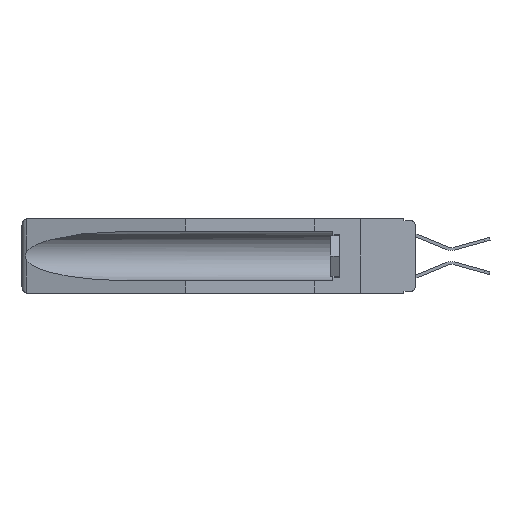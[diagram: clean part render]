
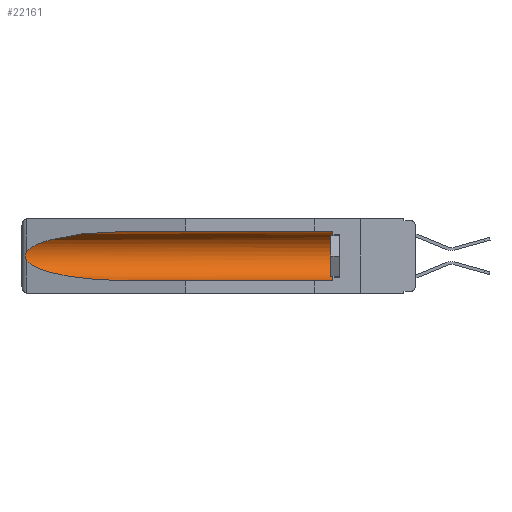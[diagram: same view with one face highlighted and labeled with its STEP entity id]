
A CAD part, left-side view. The second image highlights one B-rep face of the part: STEP entity #22161.
In plain terms, the highlighted cylindrical face has radius 2.857 mm (diameter 5.715 mm), a partial arc.
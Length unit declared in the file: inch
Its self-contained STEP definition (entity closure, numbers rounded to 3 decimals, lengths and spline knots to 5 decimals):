
#208 = ORIENTED_EDGE ( 'NONE', *, *, #10696, .T. ) ;
#1434 = CARTESIAN_POINT ( 'NONE',  ( 0.26654, 1.53092, -0.15636 ) ) ;
#1797 = EDGE_CURVE ( 'NONE', #14146, #15990, #14138, .T. ) ;
#2552 = B_SPLINE_CURVE_WITH_KNOTS ( 'NONE', 3,
 ( #2900, #11640, #1434, #8320, #16979, #10608, #3758, #6043, #16693, #10334 ),
 .UNSPECIFIED., .F., .F.,
 ( 4, 2, 2, 2, 4 ),
 ( 0., 0.00029, 0.00058, 0.00087, 0.00117 ),
 .UNSPECIFIED. ) ;
#2722 = EDGE_CURVE ( 'NONE', #16128, #4695, #17081, .T. ) ;
#2880 = AXIS2_PLACEMENT_3D ( 'NONE', #21203, #14833, #19715 ) ;
#2900 = CARTESIAN_POINT ( 'NONE',  ( 0.26537, 1.52718, -0.14972 ) ) ;
#3308 = CIRCLE ( 'NONE', #19399, 0.1125 ) ;
#3592 = CARTESIAN_POINT ( 'NONE',  ( 0.155, 1.07973, -0.059 ) ) ;
#3644 = FACE_OUTER_BOUND ( 'NONE', #17063, .T. ) ;
#3758 = CARTESIAN_POINT ( 'NONE',  ( 0.2673, 1.53269, -0.17917 ) ) ;
#4298 = CARTESIAN_POINT ( 'NONE',  ( 0.21114, 1.30732, -0.059 ) ) ;
#4695 = VERTEX_POINT ( 'NONE', #18701 ) ;
#5085 = CARTESIAN_POINT ( 'NONE',  ( 0.25451, 1.48313, -0.24835 ) ) ;
#5168 = VECTOR ( 'NONE', #14206, 39.37008 ) ;
#5821 = VERTEX_POINT ( 'NONE', #14071 ) ;
#6043 = CARTESIAN_POINT ( 'NONE',  ( 0.26655, 1.53094, -0.18657 ) ) ;
#6093 = LINE ( 'NONE', #22992, #11876 ) ;
#6508 = VERTEX_POINT ( 'NONE', #17469 ) ;
#7159 = DIRECTION ( 'NONE',  ( 0., 0., 1. ) ) ;
#7865 = LINE ( 'NONE', #25184, #5168 ) ;
#8320 = CARTESIAN_POINT ( 'NONE',  ( 0.2673, 1.5327, -0.16383 ) ) ;
#8718 = CARTESIAN_POINT ( 'NONE',  ( 0.155, 1.07973, -0.059 ) ) ;
#10334 = CARTESIAN_POINT ( 'NONE',  ( 0.26537, 1.52718, -0.19328 ) ) ;
#10608 = CARTESIAN_POINT ( 'NONE',  ( 0.2675, 1.53308, -0.17534 ) ) ;
#10696 = EDGE_CURVE ( 'NONE', #5821, #6508, #3308, .T. ) ;
#10762 = EDGE_CURVE ( 'NONE', #6508, #14146, #7865, .T. ) ;
#10884 = CYLINDRICAL_SURFACE ( 'NONE', #2880, 0.1125 ) ;
#11640 = CARTESIAN_POINT ( 'NONE',  ( 0.26597, 1.52961, -0.15275 ) ) ;
#11876 = VECTOR ( 'NONE', #21510, 39.37008 ) ;
#12680 = ORIENTED_EDGE ( 'NONE', *, *, #2722, .T. ) ;
#13232 = CARTESIAN_POINT ( 'NONE',  ( 0.26537, 1.52718, -0.14972 ) ) ;
#14071 = CARTESIAN_POINT ( 'NONE',  ( 0.155, 0.126, -0.284 ) ) ;
#14138 =( BOUNDED_CURVE ( )  B_SPLINE_CURVE ( 3, ( #8718, #4298, #24304, #21844 ),
 .UNSPECIFIED., .F., .F. ) 
 B_SPLINE_CURVE_WITH_KNOTS ( ( 4, 4 ),
 ( 4.71239, 6.08839 ),
 .UNSPECIFIED. ) 
 CURVE ( )  GEOMETRIC_REPRESENTATION_ITEM ( )  RATIONAL_B_SPLINE_CURVE ( ( 1., 0.848, 0.848, 1. ) ) 
 REPRESENTATION_ITEM ( '' )  );
#14146 = VERTEX_POINT ( 'NONE', #3592 ) ;
#14206 = DIRECTION ( 'NONE',  ( 0., 1., 0. ) ) ;
#14833 = DIRECTION ( 'NONE',  ( 0., 1., 0. ) ) ;
#15002 = EDGE_CURVE ( 'NONE', #15990, #16128, #2552, .T. ) ;
#15428 = CARTESIAN_POINT ( 'NONE',  ( 0.21114, 1.30732, -0.284 ) ) ;
#15990 = VERTEX_POINT ( 'NONE', #13232 ) ;
#16128 = VERTEX_POINT ( 'NONE', #24499 ) ;
#16693 = CARTESIAN_POINT ( 'NONE',  ( 0.26597, 1.5296, -0.19026 ) ) ;
#16979 = CARTESIAN_POINT ( 'NONE',  ( 0.2675, 1.53308, -0.16763 ) ) ;
#17063 = EDGE_LOOP ( 'NONE', ( #24952, #21673, #12680, #21898, #208, #23913 ) ) ;
#17081 =( BOUNDED_CURVE ( )  B_SPLINE_CURVE ( 3, ( #24814, #5085, #15428, #24243 ),
 .UNSPECIFIED., .F., .F. ) 
 B_SPLINE_CURVE_WITH_KNOTS ( ( 4, 4 ),
 ( 0.1948, 1.5708 ),
 .UNSPECIFIED. ) 
 CURVE ( )  GEOMETRIC_REPRESENTATION_ITEM ( )  RATIONAL_B_SPLINE_CURVE ( ( 1., 0.848, 0.848, 1. ) ) 
 REPRESENTATION_ITEM ( '' )  );
#17469 = CARTESIAN_POINT ( 'NONE',  ( 0.155, 0.126, -0.059 ) ) ;
#18184 = EDGE_CURVE ( 'NONE', #5821, #4695, #6093, .T. ) ;
#18701 = CARTESIAN_POINT ( 'NONE',  ( 0.155, 1.07973, -0.284 ) ) ;
#19399 = AXIS2_PLACEMENT_3D ( 'NONE', #20147, #26879, #7159 ) ;
#19715 = DIRECTION ( 'NONE',  ( 0., 0., 1. ) ) ;
#20147 = CARTESIAN_POINT ( 'NONE',  ( 0.155, 0.126, -0.1715 ) ) ;
#21203 = CARTESIAN_POINT ( 'NONE',  ( 0.155, -0.30754, -0.1715 ) ) ;
#21510 = DIRECTION ( 'NONE',  ( 0., 1., 0. ) ) ;
#21673 = ORIENTED_EDGE ( 'NONE', *, *, #15002, .T. ) ;
#21844 = CARTESIAN_POINT ( 'NONE',  ( 0.26537, 1.52718, -0.14972 ) ) ;
#21898 = ORIENTED_EDGE ( 'NONE', *, *, #18184, .F. ) ;
#22161 = ADVANCED_FACE ( 'NONE', ( #3644 ), #10884, .F. ) ;
#22992 = CARTESIAN_POINT ( 'NONE',  ( 0.155, -0.30754, -0.284 ) ) ;
#23913 = ORIENTED_EDGE ( 'NONE', *, *, #10762, .T. ) ;
#24243 = CARTESIAN_POINT ( 'NONE',  ( 0.155, 1.07973, -0.284 ) ) ;
#24304 = CARTESIAN_POINT ( 'NONE',  ( 0.25451, 1.48313, -0.09465 ) ) ;
#24499 = CARTESIAN_POINT ( 'NONE',  ( 0.26537, 1.52718, -0.19328 ) ) ;
#24814 = CARTESIAN_POINT ( 'NONE',  ( 0.26537, 1.52718, -0.19328 ) ) ;
#24952 = ORIENTED_EDGE ( 'NONE', *, *, #1797, .T. ) ;
#25184 = CARTESIAN_POINT ( 'NONE',  ( 0.155, -0.30754, -0.059 ) ) ;
#26879 = DIRECTION ( 'NONE',  ( 0., -1., 0. ) ) ;
